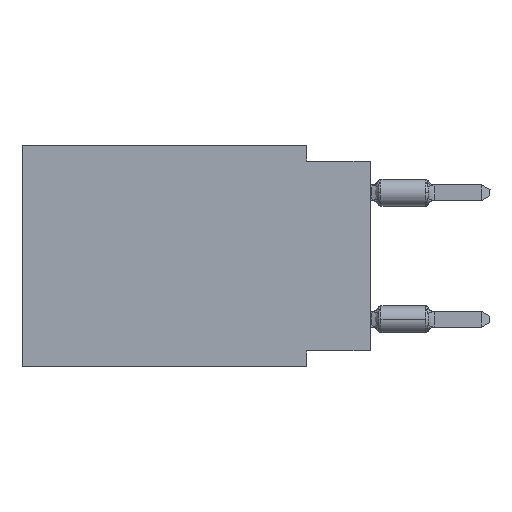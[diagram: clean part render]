
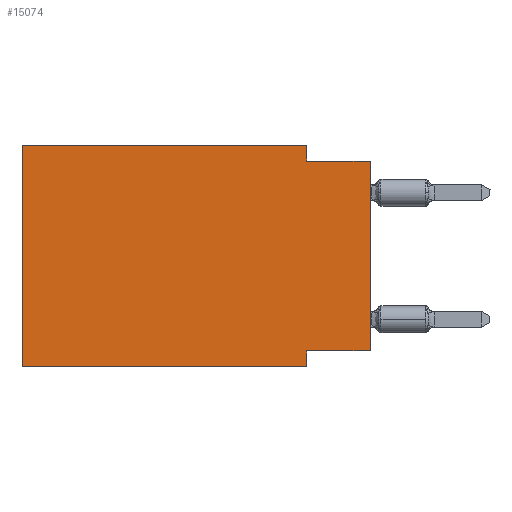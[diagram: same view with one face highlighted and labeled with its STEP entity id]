
A CAD part, left-side view. The second image highlights one B-rep face of the part: STEP entity #15074.
In plain terms, the highlighted planar face has unit normal (-1, 0, 0).
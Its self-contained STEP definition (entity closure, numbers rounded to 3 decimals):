
#244 = EDGE_CURVE ( 'NONE', #7277, #29574, #15223, .T. ) ;
#686 = CARTESIAN_POINT ( 'NONE',  ( 0., 13.97, 0. ) ) ;
#955 = DIRECTION ( 'NONE',  ( 0., 0., 1. ) ) ;
#1648 = FACE_OUTER_BOUND ( 'NONE', #35294, .T. ) ;
#1664 = ORIENTED_EDGE ( 'NONE', *, *, #244, .F. ) ;
#2731 = EDGE_CURVE ( 'NONE', #5489, #7441, #39722, .T. ) ;
#2784 = LINE ( 'NONE', #12276, #39521 ) ;
#3037 = AXIS2_PLACEMENT_3D ( 'NONE', #34549, #31439, #41580 ) ;
#3808 = ORIENTED_EDGE ( 'NONE', *, *, #2731, .F. ) ;
#5445 = VECTOR ( 'NONE', #28670, 1000. ) ;
#5489 = VERTEX_POINT ( 'NONE', #33953 ) ;
#6149 = VECTOR ( 'NONE', #14142, 1000. ) ;
#7125 = EDGE_CURVE ( 'NONE', #39263, #7277, #13478, .T. ) ;
#7277 = VERTEX_POINT ( 'NONE', #15453 ) ;
#7330 = ORIENTED_EDGE ( 'NONE', *, *, #7125, .F. ) ;
#7441 = VERTEX_POINT ( 'NONE', #11318 ) ;
#8023 = CARTESIAN_POINT ( 'NONE',  ( 0., 13.97, -8.89 ) ) ;
#8054 = CARTESIAN_POINT ( 'NONE',  ( 0., 0., -8.255 ) ) ;
#8715 = CARTESIAN_POINT ( 'NONE',  ( 0., 2.54, -0.635 ) ) ;
#10675 = CARTESIAN_POINT ( 'NONE',  ( 0., 13.97, 0. ) ) ;
#10905 = VECTOR ( 'NONE', #26061, 1000. ) ;
#11318 = CARTESIAN_POINT ( 'NONE',  ( 0., 2.54, -8.89 ) ) ;
#12276 = CARTESIAN_POINT ( 'NONE',  ( 0., 0., 0. ) ) ;
#12601 = CARTESIAN_POINT ( 'NONE',  ( 0., 2.54, -8.89 ) ) ;
#12678 = EDGE_CURVE ( 'NONE', #17451, #20840, #2784, .T. ) ;
#13478 = LINE ( 'NONE', #686, #6149 ) ;
#14142 = DIRECTION ( 'NONE',  ( 0., -1., 0. ) ) ;
#14526 = LINE ( 'NONE', #35629, #38999 ) ;
#15074 = ADVANCED_FACE ( 'NONE', ( #1648 ), #21947, .F. ) ;
#15223 = LINE ( 'NONE', #18541, #5445 ) ;
#15453 = CARTESIAN_POINT ( 'NONE',  ( 0., 2.54, 0. ) ) ;
#15636 = CARTESIAN_POINT ( 'NONE',  ( 0., 0., -0.635 ) ) ;
#16018 = CARTESIAN_POINT ( 'NONE',  ( 0., 13.97, -8.89 ) ) ;
#16029 = EDGE_CURVE ( 'NONE', #17451, #5489, #40922, .T. ) ;
#17018 = EDGE_CURVE ( 'NONE', #29988, #7441, #35672, .T. ) ;
#17451 = VERTEX_POINT ( 'NONE', #37237 ) ;
#18541 = CARTESIAN_POINT ( 'NONE',  ( 0., 2.54, 0. ) ) ;
#20840 = VERTEX_POINT ( 'NONE', #15636 ) ;
#21497 = DIRECTION ( 'NONE',  ( 0., 1., 0. ) ) ;
#21567 = VECTOR ( 'NONE', #22201, 1000. ) ;
#21947 = PLANE ( 'NONE',  #3037 ) ;
#22201 = DIRECTION ( 'NONE',  ( 0., -1., 0. ) ) ;
#26061 = DIRECTION ( 'NONE',  ( 0., 0., -1. ) ) ;
#27426 = LINE ( 'NONE', #10675, #37627 ) ;
#28670 = DIRECTION ( 'NONE',  ( 0., 0., -1. ) ) ;
#29257 = DIRECTION ( 'NONE',  ( 0., 0., 1. ) ) ;
#29488 = EDGE_CURVE ( 'NONE', #29574, #20840, #14526, .T. ) ;
#29574 = VERTEX_POINT ( 'NONE', #8715 ) ;
#29988 = VERTEX_POINT ( 'NONE', #8023 ) ;
#30770 = ORIENTED_EDGE ( 'NONE', *, *, #16029, .F. ) ;
#31081 = DIRECTION ( 'NONE',  ( 0., -1., 0. ) ) ;
#31439 = DIRECTION ( 'NONE',  ( 1., 0., 0. ) ) ;
#33283 = ORIENTED_EDGE ( 'NONE', *, *, #12678, .T. ) ;
#33390 = VECTOR ( 'NONE', #21497, 1000. ) ;
#33953 = CARTESIAN_POINT ( 'NONE',  ( 0., 2.54, -8.255 ) ) ;
#34549 = CARTESIAN_POINT ( 'NONE',  ( 0., 13.97, 0. ) ) ;
#35294 = EDGE_LOOP ( 'NONE', ( #33283, #36487, #1664, #7330, #38468, #40238, #3808, #30770 ) ) ;
#35629 = CARTESIAN_POINT ( 'NONE',  ( 0., 0., -0.635 ) ) ;
#35672 = LINE ( 'NONE', #16018, #21567 ) ;
#36487 = ORIENTED_EDGE ( 'NONE', *, *, #29488, .F. ) ;
#37237 = CARTESIAN_POINT ( 'NONE',  ( 0., 0., -8.255 ) ) ;
#37627 = VECTOR ( 'NONE', #955, 1000. ) ;
#38468 = ORIENTED_EDGE ( 'NONE', *, *, #40228, .F. ) ;
#38999 = VECTOR ( 'NONE', #31081, 1000. ) ;
#39263 = VERTEX_POINT ( 'NONE', #39944 ) ;
#39521 = VECTOR ( 'NONE', #29257, 1000. ) ;
#39722 = LINE ( 'NONE', #12601, #10905 ) ;
#39944 = CARTESIAN_POINT ( 'NONE',  ( 0., 13.97, 0. ) ) ;
#40228 = EDGE_CURVE ( 'NONE', #29988, #39263, #27426, .T. ) ;
#40238 = ORIENTED_EDGE ( 'NONE', *, *, #17018, .T. ) ;
#40922 = LINE ( 'NONE', #8054, #33390 ) ;
#41580 = DIRECTION ( 'NONE',  ( 0., 0., -1. ) ) ;
